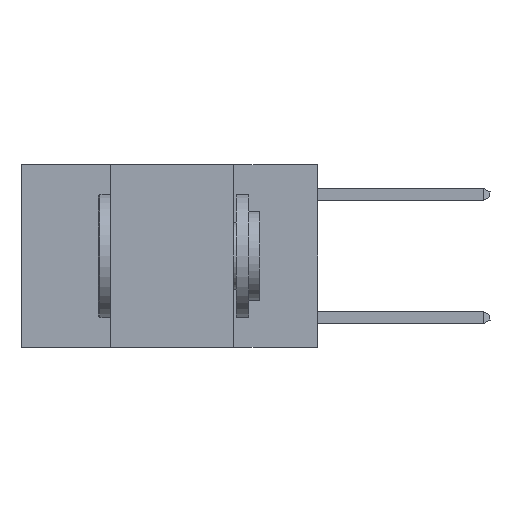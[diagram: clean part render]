
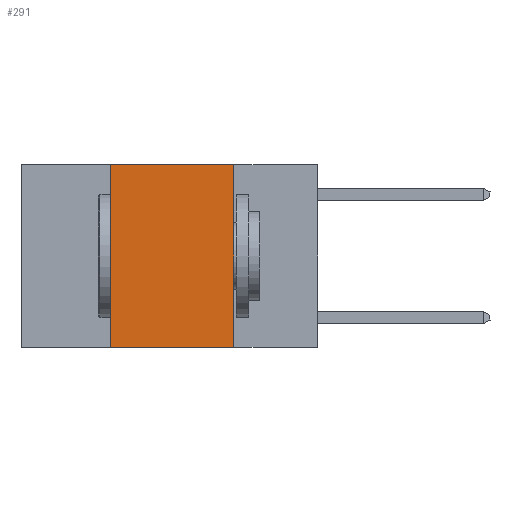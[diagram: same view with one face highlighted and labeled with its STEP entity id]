
A CAD part, left-side view. The second image highlights one B-rep face of the part: STEP entity #291.
In plain terms, the highlighted planar face has unit normal (-1, 0, 0).
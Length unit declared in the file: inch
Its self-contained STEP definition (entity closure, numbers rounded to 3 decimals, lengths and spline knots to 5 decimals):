
#291 = ADVANCED_FACE ( 'NONE', ( #21000 ), #11246, .F. ) ;
#1743 = VECTOR ( 'NONE', #2213, 39.37008 ) ;
#2213 = DIRECTION ( 'NONE',  ( 0., 0., 1. ) ) ;
#3028 = VERTEX_POINT ( 'NONE', #16322 ) ;
#3088 = CARTESIAN_POINT ( 'NONE',  ( 0., 0.6, 0. ) ) ;
#3415 = AXIS2_PLACEMENT_3D ( 'NONE', #17318, #25356, #11110 ) ;
#5223 = VECTOR ( 'NONE', #23637, 39.37008 ) ;
#5438 = CARTESIAN_POINT ( 'NONE',  ( 0., 0.17, 0. ) ) ;
#6006 = VECTOR ( 'NONE', #13960, 39.37008 ) ;
#7600 = CARTESIAN_POINT ( 'NONE',  ( 0., 0.42, 0. ) ) ;
#9012 = CARTESIAN_POINT ( 'NONE',  ( 0., 0.17, 0. ) ) ;
#9056 = LINE ( 'NONE', #3088, #14164 ) ;
#10248 = EDGE_CURVE ( 'NONE', #12789, #19190, #25487, .T. ) ;
#10950 = CARTESIAN_POINT ( 'NONE',  ( 0., 0.17, -0.37 ) ) ;
#11110 = DIRECTION ( 'NONE',  ( 0., 0., -1. ) ) ;
#11165 = DIRECTION ( 'NONE',  ( 0., -1., 0. ) ) ;
#11246 = PLANE ( 'NONE',  #3415 ) ;
#11945 = ORIENTED_EDGE ( 'NONE', *, *, #22888, .T. ) ;
#12789 = VERTEX_POINT ( 'NONE', #9012 ) ;
#13869 = ORIENTED_EDGE ( 'NONE', *, *, #10248, .F. ) ;
#13960 = DIRECTION ( 'NONE',  ( 0., -1., 0. ) ) ;
#14164 = VECTOR ( 'NONE', #11165, 39.37008 ) ;
#15010 = VERTEX_POINT ( 'NONE', #7600 ) ;
#15082 = EDGE_CURVE ( 'NONE', #15010, #12789, #9056, .T. ) ;
#15556 = EDGE_LOOP ( 'NONE', ( #13869, #20401, #23660, #11945 ) ) ;
#16322 = CARTESIAN_POINT ( 'NONE',  ( 0., 0.42, -0.37 ) ) ;
#17318 = CARTESIAN_POINT ( 'NONE',  ( 0., 0.6, 0. ) ) ;
#18098 = CARTESIAN_POINT ( 'NONE',  ( 0., 0.42, 0. ) ) ;
#19190 = VERTEX_POINT ( 'NONE', #10950 ) ;
#19809 = LINE ( 'NONE', #18098, #1743 ) ;
#20401 = ORIENTED_EDGE ( 'NONE', *, *, #15082, .F. ) ;
#21000 = FACE_OUTER_BOUND ( 'NONE', #15556, .T. ) ;
#21864 = CARTESIAN_POINT ( 'NONE',  ( 0., 0.6, -0.37 ) ) ;
#22888 = EDGE_CURVE ( 'NONE', #3028, #19190, #24222, .T. ) ;
#23637 = DIRECTION ( 'NONE',  ( 0., 0., -1. ) ) ;
#23660 = ORIENTED_EDGE ( 'NONE', *, *, #23908, .F. ) ;
#23908 = EDGE_CURVE ( 'NONE', #3028, #15010, #19809, .T. ) ;
#24222 = LINE ( 'NONE', #21864, #6006 ) ;
#25356 = DIRECTION ( 'NONE',  ( 1., 0., 0. ) ) ;
#25487 = LINE ( 'NONE', #5438, #5223 ) ;
